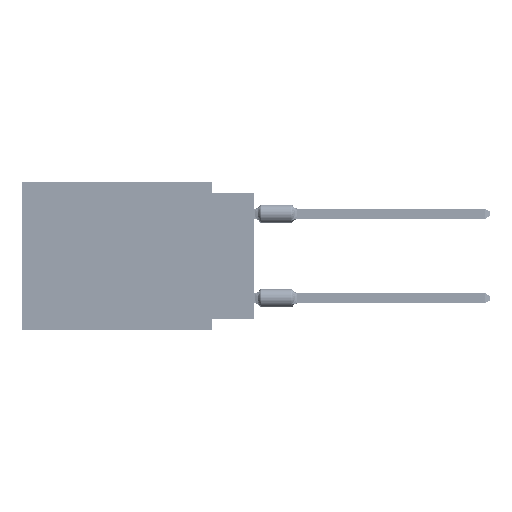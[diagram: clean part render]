
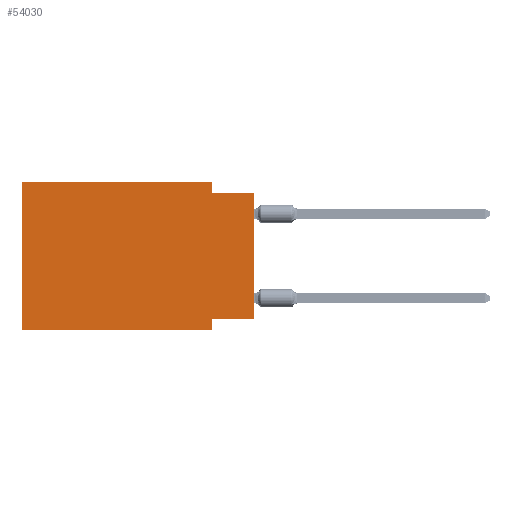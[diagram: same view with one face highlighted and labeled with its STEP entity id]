
A CAD part, left-side view. The second image highlights one B-rep face of the part: STEP entity #54030.
In plain terms, the highlighted planar face has unit normal (-1, 0, 0).
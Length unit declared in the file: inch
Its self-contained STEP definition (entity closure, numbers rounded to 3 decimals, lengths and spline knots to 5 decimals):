
#488 = LINE ( 'NONE', #97939, #12381 ) ;
#1711 = ORIENTED_EDGE ( 'NONE', *, *, #27810, .T. ) ;
#4789 = DIRECTION ( 'NONE',  ( 0., 0., -1. ) ) ;
#4861 = CARTESIAN_POINT ( 'NONE',  ( 0., 0.1, 0. ) ) ;
#4988 = VERTEX_POINT ( 'NONE', #62590 ) ;
#6834 = VERTEX_POINT ( 'NONE', #79397 ) ;
#12197 = VERTEX_POINT ( 'NONE', #95172 ) ;
#12381 = VECTOR ( 'NONE', #88928, 39.37008 ) ;
#13137 = CARTESIAN_POINT ( 'NONE',  ( 0., 0.1, -0.325 ) ) ;
#13171 = EDGE_CURVE ( 'NONE', #100165, #6834, #102422, .T. ) ;
#16372 = LINE ( 'NONE', #81496, #59806 ) ;
#17459 = EDGE_CURVE ( 'NONE', #57717, #12197, #21413, .T. ) ;
#18417 = CARTESIAN_POINT ( 'NONE',  ( 0., 0.55, 0. ) ) ;
#18976 = DIRECTION ( 'NONE',  ( 0., 1., 0. ) ) ;
#20054 = VERTEX_POINT ( 'NONE', #13137 ) ;
#20718 = LINE ( 'NONE', #4861, #55073 ) ;
#21413 = LINE ( 'NONE', #53741, #89910 ) ;
#21450 = CARTESIAN_POINT ( 'NONE',  ( 0., 0., -0.325 ) ) ;
#21816 = CARTESIAN_POINT ( 'NONE',  ( 0., 0.55, -0.35 ) ) ;
#25322 = EDGE_CURVE ( 'NONE', #6834, #4988, #20718, .T. ) ;
#27056 = PLANE ( 'NONE',  #28595 ) ;
#27810 = EDGE_CURVE ( 'NONE', #43100, #76694, #39303, .T. ) ;
#28029 = ORIENTED_EDGE ( 'NONE', *, *, #42309, .F. ) ;
#28110 = CARTESIAN_POINT ( 'NONE',  ( 0., 0.55, 0. ) ) ;
#28595 = AXIS2_PLACEMENT_3D ( 'NONE', #28110, #45060, #4789 ) ;
#29853 = DIRECTION ( 'NONE',  ( 0., -1., 0. ) ) ;
#32796 = DIRECTION ( 'NONE',  ( 0., 0., 1. ) ) ;
#33644 = ORIENTED_EDGE ( 'NONE', *, *, #49567, .F. ) ;
#36385 = VECTOR ( 'NONE', #29853, 39.37008 ) ;
#37732 = DIRECTION ( 'NONE',  ( 0., -1., 0. ) ) ;
#39303 = LINE ( 'NONE', #21816, #62153 ) ;
#40037 = VECTOR ( 'NONE', #18976, 39.37008 ) ;
#42309 = EDGE_CURVE ( 'NONE', #4988, #12197, #57416, .T. ) ;
#43099 = DIRECTION ( 'NONE',  ( 0., -1., 0. ) ) ;
#43100 = VERTEX_POINT ( 'NONE', #52745 ) ;
#45060 = DIRECTION ( 'NONE',  ( 1., 0., 0. ) ) ;
#49467 = CARTESIAN_POINT ( 'NONE',  ( 0., 0., -0.025 ) ) ;
#49567 = EDGE_CURVE ( 'NONE', #57717, #20054, #103307, .T. ) ;
#52745 = CARTESIAN_POINT ( 'NONE',  ( 0., 0.55, -0.35 ) ) ;
#52980 = FACE_OUTER_BOUND ( 'NONE', #68108, .T. ) ;
#53741 = CARTESIAN_POINT ( 'NONE',  ( 0., 0., 0. ) ) ;
#54030 = ADVANCED_FACE ( 'NONE', ( #52980 ), #27056, .F. ) ;
#55073 = VECTOR ( 'NONE', #69464, 39.37008 ) ;
#57084 = ORIENTED_EDGE ( 'NONE', *, *, #17459, .T. ) ;
#57416 = LINE ( 'NONE', #49467, #68942 ) ;
#57717 = VERTEX_POINT ( 'NONE', #21450 ) ;
#59758 = CARTESIAN_POINT ( 'NONE',  ( 0., 0., -0.325 ) ) ;
#59806 = VECTOR ( 'NONE', #32796, 39.37008 ) ;
#62153 = VECTOR ( 'NONE', #37732, 39.37008 ) ;
#62590 = CARTESIAN_POINT ( 'NONE',  ( 0., 0.1, -0.025 ) ) ;
#63329 = EDGE_CURVE ( 'NONE', #20054, #76694, #488, .T. ) ;
#68108 = EDGE_LOOP ( 'NONE', ( #57084, #28029, #73610, #75153, #81177, #1711, #87429, #33644 ) ) ;
#68942 = VECTOR ( 'NONE', #43099, 39.37008 ) ;
#69464 = DIRECTION ( 'NONE',  ( 0., 0., -1. ) ) ;
#71341 = EDGE_CURVE ( 'NONE', #43100, #100165, #16372, .T. ) ;
#73610 = ORIENTED_EDGE ( 'NONE', *, *, #25322, .F. ) ;
#75153 = ORIENTED_EDGE ( 'NONE', *, *, #13171, .F. ) ;
#76694 = VERTEX_POINT ( 'NONE', #86279 ) ;
#79397 = CARTESIAN_POINT ( 'NONE',  ( 0., 0.1, 0. ) ) ;
#81177 = ORIENTED_EDGE ( 'NONE', *, *, #71341, .F. ) ;
#81496 = CARTESIAN_POINT ( 'NONE',  ( 0., 0.55, 0. ) ) ;
#86279 = CARTESIAN_POINT ( 'NONE',  ( 0., 0.1, -0.35 ) ) ;
#86541 = DIRECTION ( 'NONE',  ( 0., 0., 1. ) ) ;
#87429 = ORIENTED_EDGE ( 'NONE', *, *, #63329, .F. ) ;
#87541 = CARTESIAN_POINT ( 'NONE',  ( 0., 0.55, 0. ) ) ;
#88928 = DIRECTION ( 'NONE',  ( 0., 0., -1. ) ) ;
#89910 = VECTOR ( 'NONE', #86541, 39.37008 ) ;
#95172 = CARTESIAN_POINT ( 'NONE',  ( 0., 0., -0.025 ) ) ;
#97939 = CARTESIAN_POINT ( 'NONE',  ( 0., 0.1, -0.35 ) ) ;
#100165 = VERTEX_POINT ( 'NONE', #18417 ) ;
#102422 = LINE ( 'NONE', #87541, #36385 ) ;
#103307 = LINE ( 'NONE', #59758, #40037 ) ;
